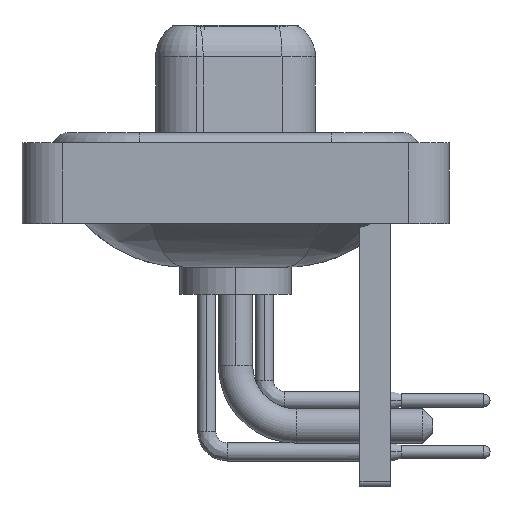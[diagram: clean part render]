
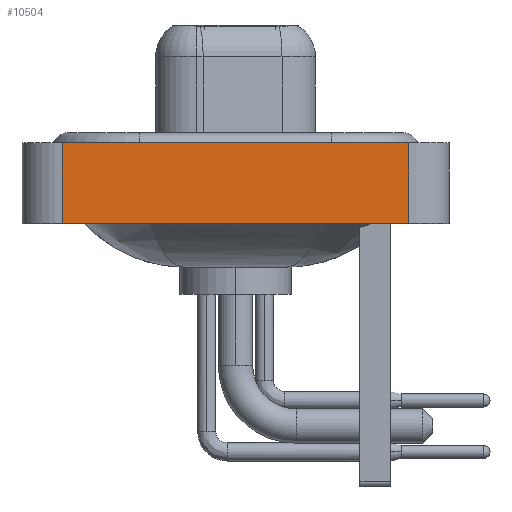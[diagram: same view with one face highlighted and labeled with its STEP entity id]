
A CAD part, left-side view. The second image highlights one B-rep face of the part: STEP entity #10504.
In plain terms, the highlighted planar face has unit normal (-1, 0, 0).
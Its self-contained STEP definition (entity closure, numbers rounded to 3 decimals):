
#40 = DIRECTION ( 'NONE',  ( 0., 0., 1. ) ) ;
#105 = ORIENTED_EDGE ( 'NONE', *, *, #7724, .T. ) ;
#135 = VECTOR ( 'NONE', #10469, 1000. ) ;
#145 = CARTESIAN_POINT ( 'NONE',  ( -7.3, -8.55, -3.6 ) ) ;
#608 = CARTESIAN_POINT ( 'NONE',  ( -7.3, 8.55, 0.4 ) ) ;
#687 = CARTESIAN_POINT ( 'NONE',  ( -7.3, 8.55, -3.6 ) ) ;
#1068 = DIRECTION ( 'NONE',  ( 0., 0., 1. ) ) ;
#3727 = CARTESIAN_POINT ( 'NONE',  ( -7.3, -8.55, -3.6 ) ) ;
#4418 = CARTESIAN_POINT ( 'NONE',  ( -7.3, 8.55, -3.6 ) ) ;
#6785 = ORIENTED_EDGE ( 'NONE', *, *, #21435, .F. ) ;
#7235 = EDGE_LOOP ( 'NONE', ( #105, #9617, #6785, #8795 ) ) ;
#7342 = VECTOR ( 'NONE', #18313, 1000. ) ;
#7724 = EDGE_CURVE ( 'NONE', #13373, #9838, #13305, .T. ) ;
#8795 = ORIENTED_EDGE ( 'NONE', *, *, #15200, .T. ) ;
#9617 = ORIENTED_EDGE ( 'NONE', *, *, #12669, .F. ) ;
#9838 = VERTEX_POINT ( 'NONE', #18182 ) ;
#10469 = DIRECTION ( 'NONE',  ( 0., -1., 0. ) ) ;
#10504 = ADVANCED_FACE ( 'NONE', ( #10648 ), #17292, .T. ) ;
#10648 = FACE_OUTER_BOUND ( 'NONE', #7235, .T. ) ;
#12026 = LINE ( 'NONE', #15179, #7342 ) ;
#12436 = DIRECTION ( 'NONE',  ( 0., 0., 1. ) ) ;
#12669 = EDGE_CURVE ( 'NONE', #20215, #9838, #12026, .T. ) ;
#13305 = LINE ( 'NONE', #145, #21294 ) ;
#13373 = VERTEX_POINT ( 'NONE', #13479 ) ;
#13479 = CARTESIAN_POINT ( 'NONE',  ( -7.3, -8.55, -3.6 ) ) ;
#15179 = CARTESIAN_POINT ( 'NONE',  ( -7.3, -8.55, 0.4 ) ) ;
#15200 = EDGE_CURVE ( 'NONE', #17067, #13373, #16901, .T. ) ;
#16901 = LINE ( 'NONE', #3727, #135 ) ;
#17067 = VERTEX_POINT ( 'NONE', #4418 ) ;
#17292 = PLANE ( 'NONE',  #19062 ) ;
#18182 = CARTESIAN_POINT ( 'NONE',  ( -7.3, -8.55, 0.4 ) ) ;
#18313 = DIRECTION ( 'NONE',  ( 0., -1., 0. ) ) ;
#19062 = AXIS2_PLACEMENT_3D ( 'NONE', #19111, #19315, #1068 ) ;
#19111 = CARTESIAN_POINT ( 'NONE',  ( -7.3, -8.55, -3.6 ) ) ;
#19315 = DIRECTION ( 'NONE',  ( -1., 0., 0. ) ) ;
#20215 = VERTEX_POINT ( 'NONE', #608 ) ;
#20440 = LINE ( 'NONE', #687, #21282 ) ;
#21282 = VECTOR ( 'NONE', #12436, 1000. ) ;
#21294 = VECTOR ( 'NONE', #40, 1000. ) ;
#21435 = EDGE_CURVE ( 'NONE', #17067, #20215, #20440, .T. ) ;
